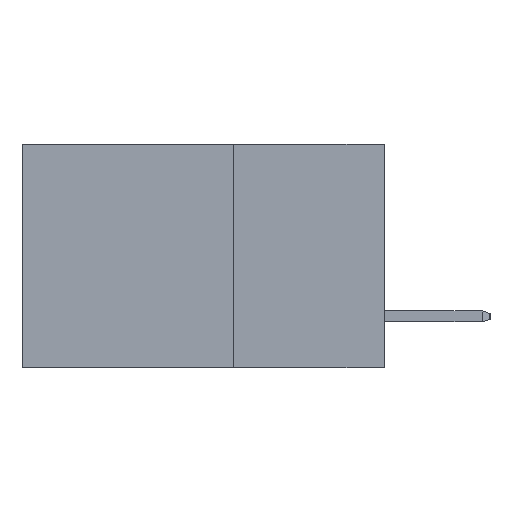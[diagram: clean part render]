
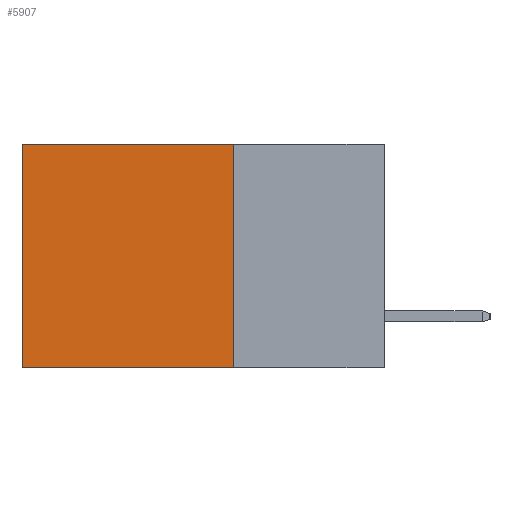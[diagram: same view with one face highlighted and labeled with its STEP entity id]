
A CAD part, left-side view. The second image highlights one B-rep face of the part: STEP entity #5907.
In plain terms, the highlighted planar face has unit normal (-1, 0, 0).
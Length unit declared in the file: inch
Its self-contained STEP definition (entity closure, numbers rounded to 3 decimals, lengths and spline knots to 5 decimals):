
#643 = ORIENTED_EDGE ( 'NONE', *, *, #9747, .T. ) ;
#898 = EDGE_CURVE ( 'NONE', #14666, #3610, #14575, .T. ) ;
#1670 = CARTESIAN_POINT ( 'NONE',  ( 0.298, 0.6, 0. ) ) ;
#1807 = ORIENTED_EDGE ( 'NONE', *, *, #898, .T. ) ;
#2501 = LINE ( 'NONE', #4749, #8684 ) ;
#2522 = LINE ( 'NONE', #15035, #12686 ) ;
#2741 = EDGE_CURVE ( 'NONE', #14666, #12212, #2522, .T. ) ;
#2851 = CARTESIAN_POINT ( 'NONE',  ( 0.298, 0.25, 0. ) ) ;
#3610 = VERTEX_POINT ( 'NONE', #1670 ) ;
#3881 = LINE ( 'NONE', #14484, #6954 ) ;
#4414 = VECTOR ( 'NONE', #15966, 39.37008 ) ;
#4749 = CARTESIAN_POINT ( 'NONE',  ( 0.298, 0.25, -0.37 ) ) ;
#5122 = DIRECTION ( 'NONE',  ( 1., 0., 0. ) ) ;
#5907 = ADVANCED_FACE ( 'NONE', ( #9843 ), #13111, .F. ) ;
#5924 = DIRECTION ( 'NONE',  ( 0., 0., -1. ) ) ;
#6060 = EDGE_LOOP ( 'NONE', ( #643, #10095, #10783, #1807 ) ) ;
#6954 = VECTOR ( 'NONE', #7863, 39.37008 ) ;
#7863 = DIRECTION ( 'NONE',  ( 0., 0., -1. ) ) ;
#8684 = VECTOR ( 'NONE', #15342, 39.37008 ) ;
#8946 = CARTESIAN_POINT ( 'NONE',  ( 0.298, 0.25, -0.37 ) ) ;
#9085 = CARTESIAN_POINT ( 'NONE',  ( 0.298, 0.25, 0. ) ) ;
#9747 = EDGE_CURVE ( 'NONE', #3610, #10347, #3881, .T. ) ;
#9843 = FACE_OUTER_BOUND ( 'NONE', #6060, .T. ) ;
#10095 = ORIENTED_EDGE ( 'NONE', *, *, #12771, .F. ) ;
#10230 = CARTESIAN_POINT ( 'NONE',  ( 0.298, 0.6, -0.37 ) ) ;
#10347 = VERTEX_POINT ( 'NONE', #10230 ) ;
#10783 = ORIENTED_EDGE ( 'NONE', *, *, #2741, .F. ) ;
#11119 = CARTESIAN_POINT ( 'NONE',  ( 0.298, 0.25, 0. ) ) ;
#11156 = AXIS2_PLACEMENT_3D ( 'NONE', #9085, #5122, #14414 ) ;
#12212 = VERTEX_POINT ( 'NONE', #8946 ) ;
#12686 = VECTOR ( 'NONE', #5924, 39.37008 ) ;
#12771 = EDGE_CURVE ( 'NONE', #12212, #10347, #2501, .T. ) ;
#13111 = PLANE ( 'NONE',  #11156 ) ;
#14414 = DIRECTION ( 'NONE',  ( 0., 0., -1. ) ) ;
#14484 = CARTESIAN_POINT ( 'NONE',  ( 0.298, 0.6, 0. ) ) ;
#14575 = LINE ( 'NONE', #11119, #4414 ) ;
#14666 = VERTEX_POINT ( 'NONE', #2851 ) ;
#15035 = CARTESIAN_POINT ( 'NONE',  ( 0.298, 0.25, 0. ) ) ;
#15342 = DIRECTION ( 'NONE',  ( 0., 1., 0. ) ) ;
#15966 = DIRECTION ( 'NONE',  ( 0., 1., 0. ) ) ;
